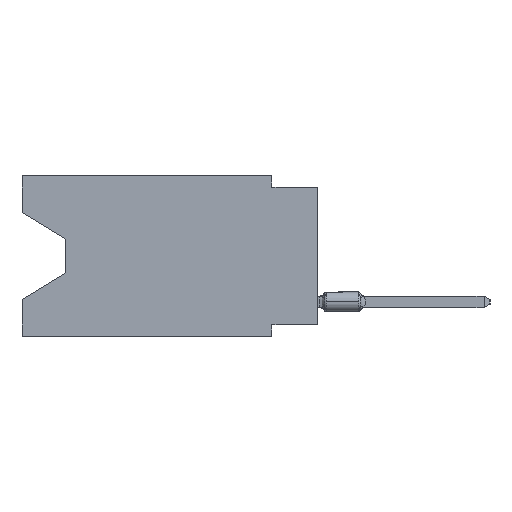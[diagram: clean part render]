
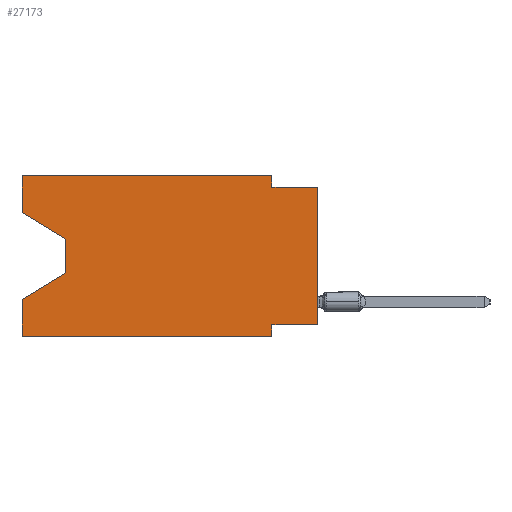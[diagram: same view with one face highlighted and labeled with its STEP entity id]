
A CAD part, left-side view. The second image highlights one B-rep face of the part: STEP entity #27173.
In plain terms, the highlighted planar face has unit normal (-1, 0, 0).
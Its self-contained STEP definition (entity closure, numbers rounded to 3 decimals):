
#648 = VECTOR ( 'NONE', #26210, 1000. ) ;
#931 = ORIENTED_EDGE ( 'NONE', *, *, #31947, .F. ) ;
#1872 = ORIENTED_EDGE ( 'NONE', *, *, #16435, .T. ) ;
#2098 = CARTESIAN_POINT ( 'NONE',  ( 0., 13.97, -5.385 ) ) ;
#2274 = CARTESIAN_POINT ( 'NONE',  ( 0., 2.54, -0.635 ) ) ;
#2328 = CARTESIAN_POINT ( 'NONE',  ( 0., 16.383, 0. ) ) ;
#2384 = VERTEX_POINT ( 'NONE', #24190 ) ;
#2496 = PLANE ( 'NONE',  #12570 ) ;
#3079 = CARTESIAN_POINT ( 'NONE',  ( 0., 2.54, 0. ) ) ;
#3228 = CARTESIAN_POINT ( 'NONE',  ( 0., 16.383, -2.038 ) ) ;
#3592 = LINE ( 'NONE', #6006, #34078 ) ;
#3862 = DIRECTION ( 'NONE',  ( 0., 0., -1. ) ) ;
#3937 = VECTOR ( 'NONE', #3862, 1000. ) ;
#4205 = LINE ( 'NONE', #18683, #5569 ) ;
#4350 = ORIENTED_EDGE ( 'NONE', *, *, #5512, .T. ) ;
#4432 = VECTOR ( 'NONE', #27619, 1000. ) ;
#5155 = VERTEX_POINT ( 'NONE', #31815 ) ;
#5289 = LINE ( 'NONE', #2328, #12583 ) ;
#5411 = CARTESIAN_POINT ( 'NONE',  ( 0., 16.383, -6.852 ) ) ;
#5512 = EDGE_CURVE ( 'NONE', #21258, #2384, #26019, .T. ) ;
#5534 = CARTESIAN_POINT ( 'NONE',  ( 0., 0., 0. ) ) ;
#5569 = VECTOR ( 'NONE', #15520, 1000. ) ;
#5814 = LINE ( 'NONE', #11917, #26251 ) ;
#6006 = CARTESIAN_POINT ( 'NONE',  ( 0., 16.383, -2.038 ) ) ;
#6758 = EDGE_CURVE ( 'NONE', #10828, #26731, #5289, .T. ) ;
#7473 = LINE ( 'NONE', #2098, #22843 ) ;
#7652 = DIRECTION ( 'NONE',  ( 0., 0.855, -0.519 ) ) ;
#8062 = DIRECTION ( 'NONE',  ( 0., 0., -1. ) ) ;
#8281 = ORIENTED_EDGE ( 'NONE', *, *, #12555, .T. ) ;
#9857 = EDGE_CURVE ( 'NONE', #21176, #19088, #24844, .T. ) ;
#10046 = EDGE_CURVE ( 'NONE', #26731, #26879, #4205, .T. ) ;
#10369 = LINE ( 'NONE', #33727, #4432 ) ;
#10535 = EDGE_CURVE ( 'NONE', #21258, #11220, #10369, .T. ) ;
#10828 = VERTEX_POINT ( 'NONE', #3228 ) ;
#10842 = FACE_OUTER_BOUND ( 'NONE', #26104, .T. ) ;
#11022 = DIRECTION ( 'NONE',  ( 1., 0., 0. ) ) ;
#11220 = VERTEX_POINT ( 'NONE', #5411 ) ;
#11384 = ORIENTED_EDGE ( 'NONE', *, *, #10046, .F. ) ;
#11611 = ORIENTED_EDGE ( 'NONE', *, *, #36601, .T. ) ;
#11917 = CARTESIAN_POINT ( 'NONE',  ( 0., 0., -8.255 ) ) ;
#12000 = VECTOR ( 'NONE', #12701, 1000. ) ;
#12143 = LINE ( 'NONE', #26629, #12000 ) ;
#12409 = VECTOR ( 'NONE', #34952, 1000. ) ;
#12555 = EDGE_CURVE ( 'NONE', #10828, #17595, #3592, .T. ) ;
#12570 = AXIS2_PLACEMENT_3D ( 'NONE', #19554, #11022, #8062 ) ;
#12583 = VECTOR ( 'NONE', #19030, 1000. ) ;
#12701 = DIRECTION ( 'NONE',  ( 0., 0., -1. ) ) ;
#14543 = DIRECTION ( 'NONE',  ( 0., -0.855, -0.519 ) ) ;
#15520 = DIRECTION ( 'NONE',  ( 0., -1., 0. ) ) ;
#16435 = EDGE_CURVE ( 'NONE', #17595, #5155, #12143, .T. ) ;
#17041 = CARTESIAN_POINT ( 'NONE',  ( 0., 0., -0.635 ) ) ;
#17595 = VERTEX_POINT ( 'NONE', #22264 ) ;
#17619 = ORIENTED_EDGE ( 'NONE', *, *, #28650, .F. ) ;
#18423 = CARTESIAN_POINT ( 'NONE',  ( 0., 2.54, 0. ) ) ;
#18683 = CARTESIAN_POINT ( 'NONE',  ( 0., 16.383, 0. ) ) ;
#19030 = DIRECTION ( 'NONE',  ( 0., 0., 1. ) ) ;
#19088 = VERTEX_POINT ( 'NONE', #28054 ) ;
#19554 = CARTESIAN_POINT ( 'NONE',  ( 0., 16.383, 0. ) ) ;
#19579 = EDGE_CURVE ( 'NONE', #26960, #2384, #34481, .T. ) ;
#19781 = CARTESIAN_POINT ( 'NONE',  ( 0., 2.54, -8.255 ) ) ;
#20474 = DIRECTION ( 'NONE',  ( 0., 1., 0. ) ) ;
#20566 = CARTESIAN_POINT ( 'NONE',  ( 0., 2.54, -8.89 ) ) ;
#21161 = ORIENTED_EDGE ( 'NONE', *, *, #6758, .F. ) ;
#21176 = VERTEX_POINT ( 'NONE', #28157 ) ;
#21258 = VERTEX_POINT ( 'NONE', #32222 ) ;
#21601 = ORIENTED_EDGE ( 'NONE', *, *, #10535, .F. ) ;
#22264 = CARTESIAN_POINT ( 'NONE',  ( 0., 13.97, -3.505 ) ) ;
#22843 = VECTOR ( 'NONE', #7652, 1000. ) ;
#24091 = ORIENTED_EDGE ( 'NONE', *, *, #19579, .F. ) ;
#24154 = DIRECTION ( 'NONE',  ( 0., 0., 1. ) ) ;
#24190 = CARTESIAN_POINT ( 'NONE',  ( 0., 2.54, -8.89 ) ) ;
#24844 = LINE ( 'NONE', #5534, #31050 ) ;
#26019 = LINE ( 'NONE', #31593, #648 ) ;
#26104 = EDGE_LOOP ( 'NONE', ( #8281, #1872, #11611, #21601, #4350, #24091, #28484, #34985, #931, #17619, #11384, #21161 ) ) ;
#26210 = DIRECTION ( 'NONE',  ( 0., -1., 0. ) ) ;
#26251 = VECTOR ( 'NONE', #20474, 1000. ) ;
#26498 = VECTOR ( 'NONE', #34127, 1000. ) ;
#26629 = CARTESIAN_POINT ( 'NONE',  ( 0., 13.97, -3.505 ) ) ;
#26731 = VERTEX_POINT ( 'NONE', #30576 ) ;
#26879 = VERTEX_POINT ( 'NONE', #3079 ) ;
#26960 = VERTEX_POINT ( 'NONE', #19781 ) ;
#27173 = ADVANCED_FACE ( 'NONE', ( #10842 ), #2496, .F. ) ;
#27295 = EDGE_CURVE ( 'NONE', #21176, #26960, #5814, .T. ) ;
#27619 = DIRECTION ( 'NONE',  ( 0., 0., 1. ) ) ;
#28054 = CARTESIAN_POINT ( 'NONE',  ( 0., 0., -0.635 ) ) ;
#28157 = CARTESIAN_POINT ( 'NONE',  ( 0., 0., -8.255 ) ) ;
#28484 = ORIENTED_EDGE ( 'NONE', *, *, #27295, .F. ) ;
#28650 = EDGE_CURVE ( 'NONE', #26879, #36558, #29954, .T. ) ;
#29954 = LINE ( 'NONE', #18423, #12409 ) ;
#30576 = CARTESIAN_POINT ( 'NONE',  ( 0., 16.383, 0. ) ) ;
#31050 = VECTOR ( 'NONE', #24154, 1000. ) ;
#31167 = LINE ( 'NONE', #17041, #26498 ) ;
#31593 = CARTESIAN_POINT ( 'NONE',  ( 0., 16.383, -8.89 ) ) ;
#31815 = CARTESIAN_POINT ( 'NONE',  ( 0., 13.97, -5.385 ) ) ;
#31947 = EDGE_CURVE ( 'NONE', #36558, #19088, #31167, .T. ) ;
#32222 = CARTESIAN_POINT ( 'NONE',  ( 0., 16.383, -8.89 ) ) ;
#33727 = CARTESIAN_POINT ( 'NONE',  ( 0., 16.383, 0. ) ) ;
#34078 = VECTOR ( 'NONE', #14543, 1000. ) ;
#34127 = DIRECTION ( 'NONE',  ( 0., -1., 0. ) ) ;
#34481 = LINE ( 'NONE', #20566, #3937 ) ;
#34952 = DIRECTION ( 'NONE',  ( 0., 0., -1. ) ) ;
#34985 = ORIENTED_EDGE ( 'NONE', *, *, #9857, .T. ) ;
#36558 = VERTEX_POINT ( 'NONE', #2274 ) ;
#36601 = EDGE_CURVE ( 'NONE', #5155, #11220, #7473, .T. ) ;
